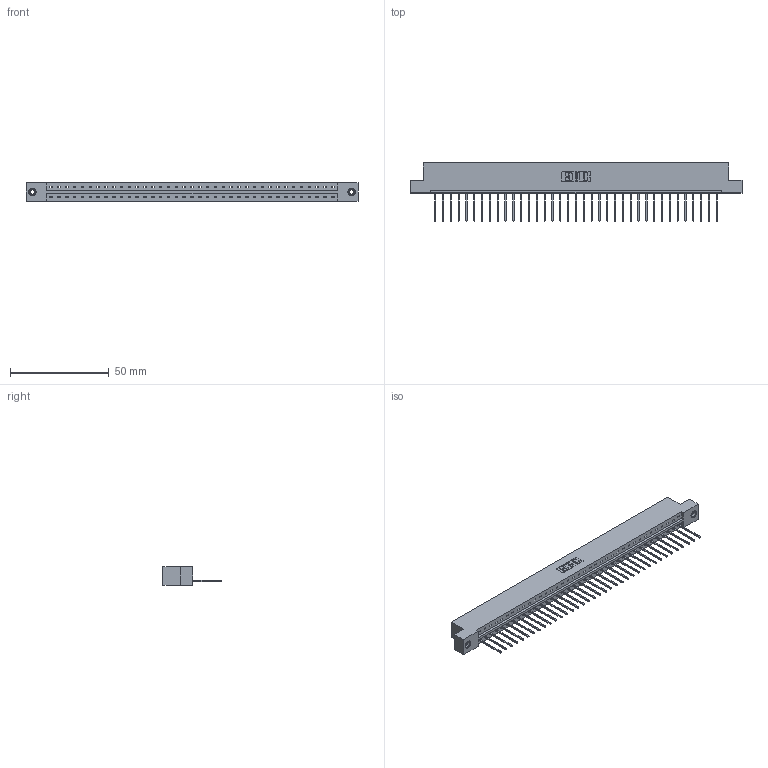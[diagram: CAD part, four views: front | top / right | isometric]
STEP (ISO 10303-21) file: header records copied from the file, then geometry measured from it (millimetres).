
FILE_DESCRIPTION (( 'STEP AP203' ), '1' );
FILE_NAME ('333-037-540-108.STEP', '2018-08-03T02:36:33', ( '' ), ( '' ), 'SwSTEP 2.0', 'SolidWorks 2016', '' );
FILE_SCHEMA (( 'CONFIG_CONTROL_DESIGN' ));
Length unit declared in the file: inch
Products named in the file (4): 333 Part_Flush - .156 Dia - TI; 345-292-001_345-293-140; 345-250-001_345-250-003-102; 333-037-540-108
Assembly tree (40 placements, depth 2):
  333-037-540-108
    333 Part_Flush - .156 Dia - TI
    345-292-001_345-293-140  x37
    345-250-001_345-250-003-102  x2
Bounding box: 168.15 x 29.47 x 9.4 mm (x, y, z)
Volume: 16921 mm3; surface area: 18675.4 mm2
Topology: 40 solids, 40 shells, 2320 faces, 6959 edges, 4582 vertices
Faces by surface type: plane 1656, cylinder 648, cone 12, torus 4
Entity records: 24470 total; most frequent: CARTESIAN_POINT 4204, ORIENTED_EDGE 4170, DIRECTION 3589, EDGE_CURVE 2085, LINE 1937, VECTOR 1937, VERTEX_POINT 1384, AXIS2_PLACEMENT_3D 826
